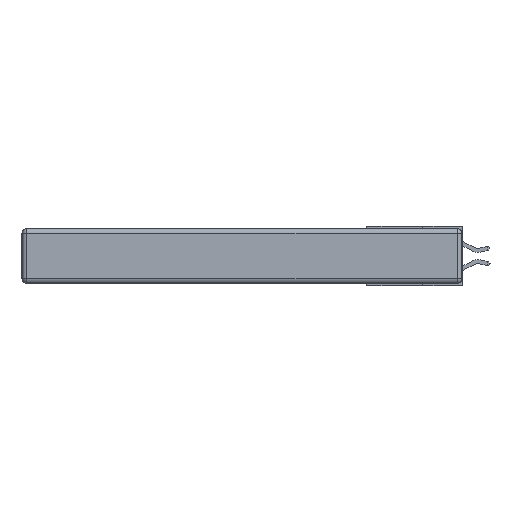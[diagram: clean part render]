
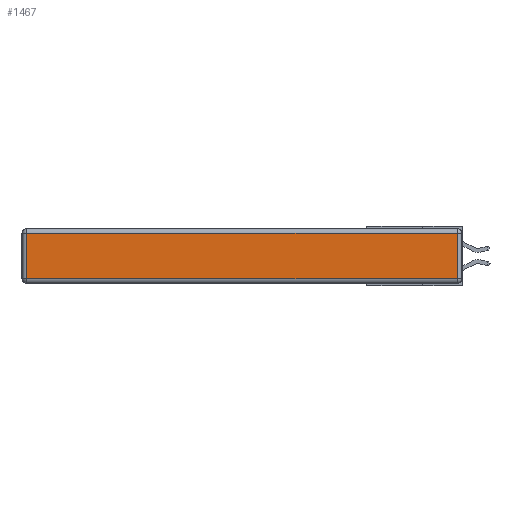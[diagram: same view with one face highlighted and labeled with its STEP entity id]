
A CAD part, left-side view. The second image highlights one B-rep face of the part: STEP entity #1467.
In plain terms, the highlighted planar face has unit normal (-1, 0, 0).
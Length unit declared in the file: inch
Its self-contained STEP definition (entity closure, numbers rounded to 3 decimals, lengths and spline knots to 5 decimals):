
#83 = CARTESIAN_POINT ( 'NONE',  ( 0., 2.75, -0.03 ) ) ;
#383 = VECTOR ( 'NONE', #26699, 39.37008 ) ;
#1467 = ADVANCED_FACE ( 'NONE', ( #24151 ), #11846, .T. ) ;
#1732 = CARTESIAN_POINT ( 'NONE',  ( 0., 0., -0.313 ) ) ;
#1738 = CARTESIAN_POINT ( 'NONE',  ( 0., 2.72, -0.03 ) ) ;
#2491 = DIRECTION ( 'NONE',  ( -1., 0., 0. ) ) ;
#2977 = LINE ( 'NONE', #21466, #25448 ) ;
#4079 = ORIENTED_EDGE ( 'NONE', *, *, #15035, .T. ) ;
#4580 = DIRECTION ( 'NONE',  ( 0., 0., 1. ) ) ;
#7841 = CARTESIAN_POINT ( 'NONE',  ( 0., 0.03, -0.03 ) ) ;
#8265 = VERTEX_POINT ( 'NONE', #7841 ) ;
#8394 = EDGE_CURVE ( 'NONE', #16721, #8265, #2977, .T. ) ;
#8859 = AXIS2_PLACEMENT_3D ( 'NONE', #9480, #2491, #4580 ) ;
#9480 = CARTESIAN_POINT ( 'NONE',  ( 0., 0., -0.343 ) ) ;
#9859 = DIRECTION ( 'NONE',  ( 0., 0., 1. ) ) ;
#11216 = VECTOR ( 'NONE', #30552, 39.37008 ) ;
#11846 = PLANE ( 'NONE',  #8859 ) ;
#14734 = ORIENTED_EDGE ( 'NONE', *, *, #8394, .T. ) ;
#15035 = EDGE_CURVE ( 'NONE', #8265, #18088, #28156, .T. ) ;
#15408 = EDGE_CURVE ( 'NONE', #22882, #16721, #25123, .T. ) ;
#15419 = EDGE_LOOP ( 'NONE', ( #16648, #14734, #4079, #26320 ) ) ;
#16121 = CARTESIAN_POINT ( 'NONE',  ( 0., 0.03, -0.313 ) ) ;
#16648 = ORIENTED_EDGE ( 'NONE', *, *, #15408, .T. ) ;
#16721 = VERTEX_POINT ( 'NONE', #16121 ) ;
#17270 = DIRECTION ( 'NONE',  ( 0., 0., -1. ) ) ;
#18088 = VERTEX_POINT ( 'NONE', #1738 ) ;
#19627 = VECTOR ( 'NONE', #17270, 39.37008 ) ;
#20723 = CARTESIAN_POINT ( 'NONE',  ( 0., 2.72, -0.313 ) ) ;
#21466 = CARTESIAN_POINT ( 'NONE',  ( 0., 0.03, -0.343 ) ) ;
#22882 = VERTEX_POINT ( 'NONE', #20723 ) ;
#24151 = FACE_OUTER_BOUND ( 'NONE', #15419, .T. ) ;
#24258 = CARTESIAN_POINT ( 'NONE',  ( 0., 2.72, -0.343 ) ) ;
#24888 = EDGE_CURVE ( 'NONE', #18088, #22882, #30929, .T. ) ;
#25123 = LINE ( 'NONE', #1732, #11216 ) ;
#25448 = VECTOR ( 'NONE', #9859, 39.37008 ) ;
#26320 = ORIENTED_EDGE ( 'NONE', *, *, #24888, .T. ) ;
#26699 = DIRECTION ( 'NONE',  ( 0., 1., 0. ) ) ;
#28156 = LINE ( 'NONE', #83, #383 ) ;
#30552 = DIRECTION ( 'NONE',  ( 0., -1., 0. ) ) ;
#30929 = LINE ( 'NONE', #24258, #19627 ) ;
